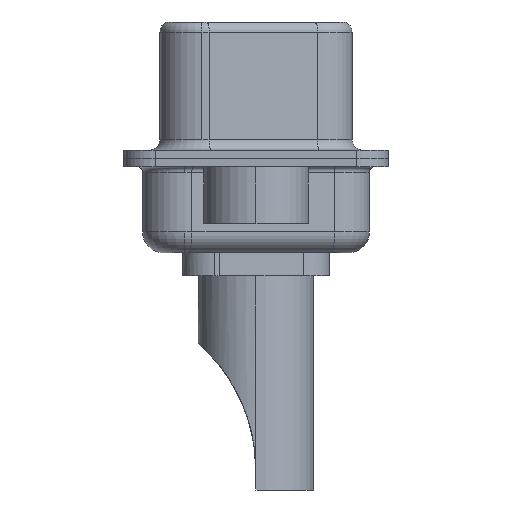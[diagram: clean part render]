
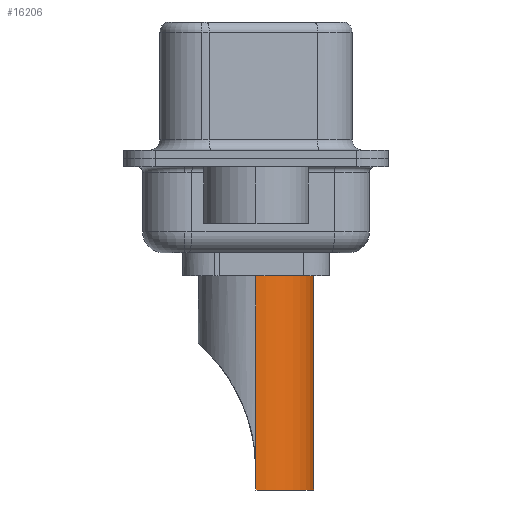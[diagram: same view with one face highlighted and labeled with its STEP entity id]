
A CAD part, left-side view. The second image highlights one B-rep face of the part: STEP entity #16206.
In plain terms, the highlighted cylindrical face has radius 2.75 mm (diameter 5.5 mm), a partial arc.
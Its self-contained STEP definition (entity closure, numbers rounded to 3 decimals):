
#470 = DIRECTION ( 'NONE',  ( 0., 0., -1. ) ) ;
#610 = EDGE_CURVE ( 'NONE', #2379, #8679, #6130, .T. ) ;
#1236 = VECTOR ( 'NONE', #18508, 1000. ) ;
#1405 = VERTEX_POINT ( 'NONE', #3136 ) ;
#2102 = DIRECTION ( 'NONE',  ( 0., 0., 1. ) ) ;
#2113 = EDGE_CURVE ( 'NONE', #3090, #9980, #16781, .T. ) ;
#2134 = CARTESIAN_POINT ( 'NONE',  ( 2.75, 0., -8.7 ) ) ;
#2322 = LINE ( 'NONE', #13340, #16385 ) ;
#2379 = VERTEX_POINT ( 'NONE', #12119 ) ;
#3002 = DIRECTION ( 'NONE',  ( 0., 0., 1. ) ) ;
#3090 = VERTEX_POINT ( 'NONE', #3621 ) ;
#3136 = CARTESIAN_POINT ( 'NONE',  ( 2.75, 0., -7.764 ) ) ;
#3621 = CARTESIAN_POINT ( 'NONE',  ( -2.75, 0., -7.764 ) ) ;
#5198 = CARTESIAN_POINT ( 'NONE',  ( -2.75, 0., -8.7 ) ) ;
#5642 = DIRECTION ( 'NONE',  ( 0., 0., 1. ) ) ;
#6130 = CIRCLE ( 'NONE', #12165, 2.75 ) ;
#7252 = CARTESIAN_POINT ( 'NONE',  ( -2.75, 0., 1.5 ) ) ;
#8007 = EDGE_CURVE ( 'NONE', #1405, #8679, #18409, .T. ) ;
#8679 = VERTEX_POINT ( 'NONE', #2134 ) ;
#9035 = CYLINDRICAL_SURFACE ( 'NONE', #14608, 2.75 ) ;
#9284 = ORIENTED_EDGE ( 'NONE', *, *, #18570, .T. ) ;
#9369 = ORIENTED_EDGE ( 'NONE', *, *, #15097, .T. ) ;
#9632 = CARTESIAN_POINT ( 'NONE',  ( 0., 0., 1.5 ) ) ;
#9683 = ORIENTED_EDGE ( 'NONE', *, *, #13230, .F. ) ;
#9980 = VERTEX_POINT ( 'NONE', #7252 ) ;
#11613 = AXIS2_PLACEMENT_3D ( 'NONE', #9632, #2102, #18821 ) ;
#11996 = CARTESIAN_POINT ( 'NONE',  ( 2.75, 0., -8.7 ) ) ;
#12119 = CARTESIAN_POINT ( 'NONE',  ( -2.75, 0., -8.7 ) ) ;
#12165 = AXIS2_PLACEMENT_3D ( 'NONE', #12263, #3002, #16790 ) ;
#12263 = CARTESIAN_POINT ( 'NONE',  ( 0., 0., -8.7 ) ) ;
#13208 = ORIENTED_EDGE ( 'NONE', *, *, #610, .T. ) ;
#13230 = EDGE_CURVE ( 'NONE', #9980, #14762, #17971, .T. ) ;
#13299 = ORIENTED_EDGE ( 'NONE', *, *, #2113, .F. ) ;
#13340 = CARTESIAN_POINT ( 'NONE',  ( 2.75, 0., 4.234 ) ) ;
#13403 = CARTESIAN_POINT ( 'NONE',  ( -2.75, 0., 4.234 ) ) ;
#13617 = DIRECTION ( 'NONE',  ( 1., 0., 0. ) ) ;
#13741 = CARTESIAN_POINT ( 'NONE',  ( 2.75, 0., 1.5 ) ) ;
#13866 = EDGE_LOOP ( 'NONE', ( #13299, #9369, #13208, #15388, #9284, #9683 ) ) ;
#13919 = LINE ( 'NONE', #5198, #16062 ) ;
#14608 = AXIS2_PLACEMENT_3D ( 'NONE', #16957, #16750, #13617 ) ;
#14762 = VERTEX_POINT ( 'NONE', #13741 ) ;
#15097 = EDGE_CURVE ( 'NONE', #3090, #2379, #13919, .T. ) ;
#15388 = ORIENTED_EDGE ( 'NONE', *, *, #8007, .F. ) ;
#16062 = VECTOR ( 'NONE', #470, 1000. ) ;
#16206 = ADVANCED_FACE ( 'NONE', ( #17862 ), #9035, .T. ) ;
#16385 = VECTOR ( 'NONE', #18584, 1000. ) ;
#16750 = DIRECTION ( 'NONE',  ( 0., 0., 1. ) ) ;
#16781 = LINE ( 'NONE', #13403, #17312 ) ;
#16790 = DIRECTION ( 'NONE',  ( 1., 0., 0. ) ) ;
#16957 = CARTESIAN_POINT ( 'NONE',  ( 0., 0., 4.234 ) ) ;
#17312 = VECTOR ( 'NONE', #5642, 1000. ) ;
#17862 = FACE_OUTER_BOUND ( 'NONE', #13866, .T. ) ;
#17971 = CIRCLE ( 'NONE', #11613, 2.75 ) ;
#18409 = LINE ( 'NONE', #11996, #1236 ) ;
#18508 = DIRECTION ( 'NONE',  ( 0., 0., -1. ) ) ;
#18570 = EDGE_CURVE ( 'NONE', #1405, #14762, #2322, .T. ) ;
#18584 = DIRECTION ( 'NONE',  ( 0., 0., 1. ) ) ;
#18821 = DIRECTION ( 'NONE',  ( 1., 0., 0. ) ) ;
